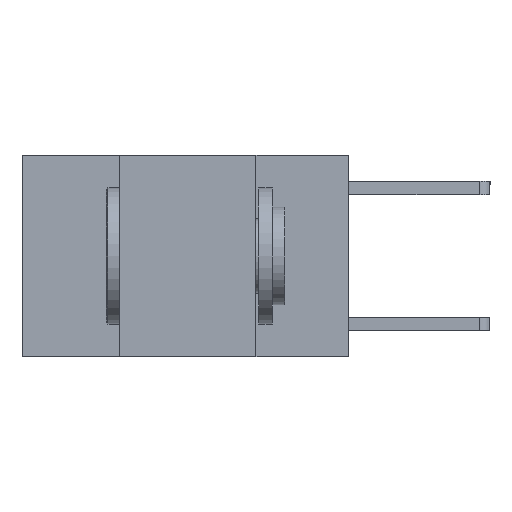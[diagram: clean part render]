
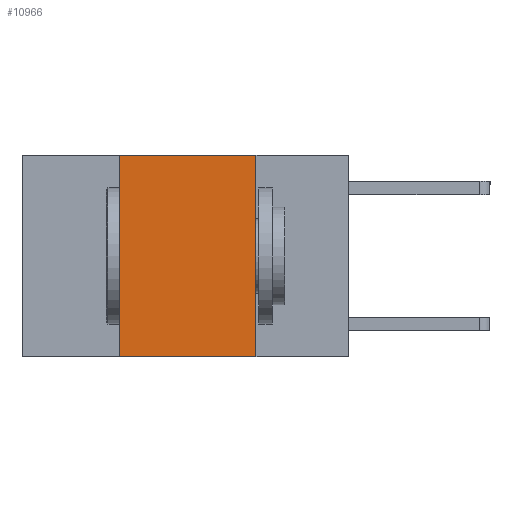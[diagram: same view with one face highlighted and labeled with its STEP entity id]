
A CAD part, left-side view. The second image highlights one B-rep face of the part: STEP entity #10966.
In plain terms, the highlighted planar face has unit normal (-1, 0, 0).
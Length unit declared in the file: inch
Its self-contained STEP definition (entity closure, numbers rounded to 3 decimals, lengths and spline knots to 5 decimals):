
#1167 = CARTESIAN_POINT ( 'NONE',  ( 0., 0.17, -0.37 ) ) ;
#1192 = LINE ( 'NONE', #10249, #9149 ) ;
#1716 = DIRECTION ( 'NONE',  ( 0., 0., -1. ) ) ;
#2371 = CARTESIAN_POINT ( 'NONE',  ( 0., 0.42, -0.37 ) ) ;
#2572 = DIRECTION ( 'NONE',  ( 0., -1., 0. ) ) ;
#2649 = DIRECTION ( 'NONE',  ( 1., 0., 0. ) ) ;
#2938 = EDGE_CURVE ( 'NONE', #4158, #8622, #1192, .T. ) ;
#3137 = CARTESIAN_POINT ( 'NONE',  ( 0., 0.17, 0. ) ) ;
#3257 = CARTESIAN_POINT ( 'NONE',  ( 0., 0.42, 0. ) ) ;
#4158 = VERTEX_POINT ( 'NONE', #4906 ) ;
#4855 = EDGE_CURVE ( 'NONE', #7460, #9904, #9633, .T. ) ;
#4906 = CARTESIAN_POINT ( 'NONE',  ( 0., 0.42, 0. ) ) ;
#5056 = VECTOR ( 'NONE', #11182, 39.37008 ) ;
#5200 = EDGE_LOOP ( 'NONE', ( #8413, #6974, #10750, #8560 ) ) ;
#5423 = EDGE_CURVE ( 'NONE', #8622, #9904, #5875, .T. ) ;
#5424 = CARTESIAN_POINT ( 'NONE',  ( 0., 0.6, 0. ) ) ;
#5776 = DIRECTION ( 'NONE',  ( 0., -1., 0. ) ) ;
#5875 = LINE ( 'NONE', #8353, #5056 ) ;
#6803 = VECTOR ( 'NONE', #2572, 39.37008 ) ;
#6857 = AXIS2_PLACEMENT_3D ( 'NONE', #5424, #2649, #1716 ) ;
#6974 = ORIENTED_EDGE ( 'NONE', *, *, #2938, .F. ) ;
#7303 = EDGE_CURVE ( 'NONE', #7460, #4158, #10391, .T. ) ;
#7460 = VERTEX_POINT ( 'NONE', #2371 ) ;
#7694 = DIRECTION ( 'NONE',  ( 0., 0., 1. ) ) ;
#8353 = CARTESIAN_POINT ( 'NONE',  ( 0., 0.17, 0. ) ) ;
#8413 = ORIENTED_EDGE ( 'NONE', *, *, #5423, .F. ) ;
#8560 = ORIENTED_EDGE ( 'NONE', *, *, #4855, .T. ) ;
#8622 = VERTEX_POINT ( 'NONE', #3137 ) ;
#8840 = FACE_OUTER_BOUND ( 'NONE', #5200, .T. ) ;
#9149 = VECTOR ( 'NONE', #5776, 39.37008 ) ;
#9293 = VECTOR ( 'NONE', #7694, 39.37008 ) ;
#9633 = LINE ( 'NONE', #9760, #6803 ) ;
#9760 = CARTESIAN_POINT ( 'NONE',  ( 0., 0.6, -0.37 ) ) ;
#9892 = PLANE ( 'NONE',  #6857 ) ;
#9904 = VERTEX_POINT ( 'NONE', #1167 ) ;
#10249 = CARTESIAN_POINT ( 'NONE',  ( 0., 0.6, 0. ) ) ;
#10391 = LINE ( 'NONE', #3257, #9293 ) ;
#10750 = ORIENTED_EDGE ( 'NONE', *, *, #7303, .F. ) ;
#10966 = ADVANCED_FACE ( 'NONE', ( #8840 ), #9892, .F. ) ;
#11182 = DIRECTION ( 'NONE',  ( 0., 0., -1. ) ) ;
